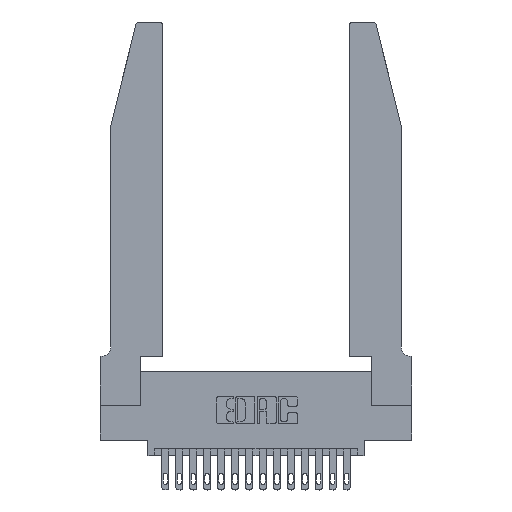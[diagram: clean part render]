
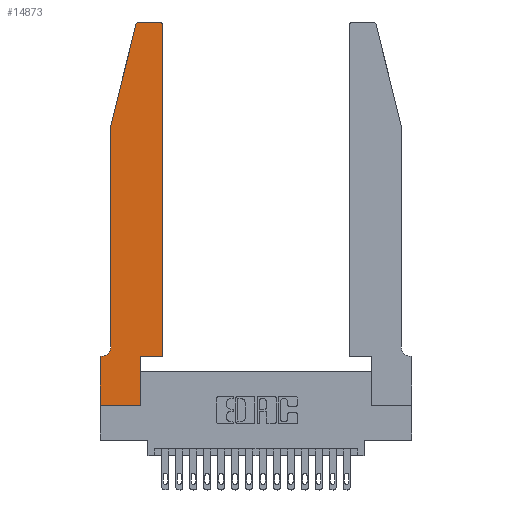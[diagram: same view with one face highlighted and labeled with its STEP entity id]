
A CAD part, top view. The second image highlights one B-rep face of the part: STEP entity #14873.
In plain terms, the highlighted planar face has unit normal (0, 0, 1).
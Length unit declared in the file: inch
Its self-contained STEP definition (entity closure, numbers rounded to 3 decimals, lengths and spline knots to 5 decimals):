
#14 = ORIENTED_EDGE ( 'NONE', *, *, #12326, .T. ) ;
#143 = LINE ( 'NONE', #4160, #15721 ) ;
#217 = VERTEX_POINT ( 'NONE', #1713 ) ;
#735 = EDGE_CURVE ( 'NONE', #17739, #10834, #6813, .T. ) ;
#847 = VERTEX_POINT ( 'NONE', #17734 ) ;
#908 = VECTOR ( 'NONE', #5271, 39.37008 ) ;
#1430 = LINE ( 'NONE', #10283, #4965 ) ;
#1468 = VERTEX_POINT ( 'NONE', #16891 ) ;
#1713 = CARTESIAN_POINT ( 'NONE',  ( 0.2865, 0., 0.37 ) ) ;
#1727 = LINE ( 'NONE', #3205, #10289 ) ;
#2108 = ORIENTED_EDGE ( 'NONE', *, *, #10911, .T. ) ;
#2228 = CARTESIAN_POINT ( 'NONE',  ( 0.4505, 0.35, 0.37 ) ) ;
#2345 = ORIENTED_EDGE ( 'NONE', *, *, #735, .T. ) ;
#2413 = EDGE_CURVE ( 'NONE', #13488, #6220, #143, .T. ) ;
#2883 = ORIENTED_EDGE ( 'NONE', *, *, #5031, .T. ) ;
#3011 = EDGE_CURVE ( 'NONE', #11351, #13488, #18828, .T. ) ;
#3040 = EDGE_CURVE ( 'NONE', #6220, #1468, #1727, .T. ) ;
#3059 = VERTEX_POINT ( 'NONE', #13959 ) ;
#3205 = CARTESIAN_POINT ( 'NONE',  ( 0.0755, 2., 0.37 ) ) ;
#3376 = EDGE_CURVE ( 'NONE', #16136, #847, #13085, .T. ) ;
#3773 = DIRECTION ( 'NONE',  ( -1., 0., 0. ) ) ;
#3942 = DIRECTION ( 'NONE',  ( -1., 0., 0. ) ) ;
#4095 = VECTOR ( 'NONE', #14769, 39.37008 ) ;
#4160 = CARTESIAN_POINT ( 'NONE',  ( 0.0755, 2., 0.37 ) ) ;
#4263 = CARTESIAN_POINT ( 'NONE',  ( 0.0755, 2., 0.37 ) ) ;
#4267 = CARTESIAN_POINT ( 'NONE',  ( 0.2865, 0.35, 0.37 ) ) ;
#4414 = ORIENTED_EDGE ( 'NONE', *, *, #9771, .T. ) ;
#4450 = CARTESIAN_POINT ( 'NONE',  ( 0., 0., 0.37 ) ) ;
#4965 = VECTOR ( 'NONE', #17643, 39.37008 ) ;
#5031 = EDGE_CURVE ( 'NONE', #1468, #17313, #15899, .T. ) ;
#5211 = CARTESIAN_POINT ( 'NONE',  ( 0.4505, 0.35, 0.37 ) ) ;
#5271 = DIRECTION ( 'NONE',  ( 1., 0., 0. ) ) ;
#5745 = FACE_OUTER_BOUND ( 'NONE', #14162, .T. ) ;
#5766 = CARTESIAN_POINT ( 'NONE',  ( 0.4205, 2.72, 0.37 ) ) ;
#6220 = VERTEX_POINT ( 'NONE', #4263 ) ;
#6303 = DIRECTION ( 'NONE',  ( 1., 0., 0. ) ) ;
#6436 = LINE ( 'NONE', #4267, #4095 ) ;
#6813 = LINE ( 'NONE', #2228, #908 ) ;
#6867 = CARTESIAN_POINT ( 'NONE',  ( 0.25487, 2.72718, 0.37 ) ) ;
#6932 = CARTESIAN_POINT ( 'NONE',  ( 0.0055, 0.42, 0.37 ) ) ;
#7708 = VECTOR ( 'NONE', #3942, 39.37008 ) ;
#7959 = CARTESIAN_POINT ( 'NONE',  ( 0.284, 2.72, 0.37 ) ) ;
#8026 = DIRECTION ( 'NONE',  ( 0., -1., 0. ) ) ;
#8660 = DIRECTION ( 'NONE',  ( 0., 1., 0. ) ) ;
#8820 = DIRECTION ( 'NONE',  ( 0., 0., 1. ) ) ;
#8932 = VERTEX_POINT ( 'NONE', #14517 ) ;
#9090 = VECTOR ( 'NONE', #8660, 39.37008 ) ;
#9267 = CARTESIAN_POINT ( 'NONE',  ( 0.4505, 0.35, 0.37 ) ) ;
#9771 = EDGE_CURVE ( 'NONE', #3059, #217, #13580, .T. ) ;
#9833 = DIRECTION ( 'NONE',  ( 0., 0., -1. ) ) ;
#10019 = ORIENTED_EDGE ( 'NONE', *, *, #3040, .T. ) ;
#10212 = PLANE ( 'NONE',  #14861 ) ;
#10280 = DIRECTION ( 'NONE',  ( 0., 0., 1. ) ) ;
#10283 = CARTESIAN_POINT ( 'NONE',  ( 0., 0., 0.37 ) ) ;
#10289 = VECTOR ( 'NONE', #8026, 39.37008 ) ;
#10834 = VERTEX_POINT ( 'NONE', #9267 ) ;
#10911 = EDGE_CURVE ( 'NONE', #10834, #16136, #16198, .T. ) ;
#11351 = VERTEX_POINT ( 'NONE', #15103 ) ;
#11529 = DIRECTION ( 'NONE',  ( 1., 0., 0. ) ) ;
#11720 = LINE ( 'NONE', #17442, #7708 ) ;
#11787 = CARTESIAN_POINT ( 'NONE',  ( 0., 0.35, 0.37 ) ) ;
#12030 = DIRECTION ( 'NONE',  ( 1., 0., 0. ) ) ;
#12326 = EDGE_CURVE ( 'NONE', #17313, #8932, #16265, .T. ) ;
#12334 = ORIENTED_EDGE ( 'NONE', *, *, #3011, .T. ) ;
#12375 = AXIS2_PLACEMENT_3D ( 'NONE', #7959, #13832, #6303 ) ;
#13019 = EDGE_CURVE ( 'NONE', #847, #11351, #11720, .T. ) ;
#13053 = CARTESIAN_POINT ( 'NONE',  ( 0.0055, 0.35, 0.37 ) ) ;
#13057 = DIRECTION ( 'NONE',  ( -1., 0., 0. ) ) ;
#13085 = CIRCLE ( 'NONE', #15807, 0.03 ) ;
#13112 = VECTOR ( 'NONE', #12030, 39.37008 ) ;
#13351 = DIRECTION ( 'NONE',  ( 1., 0., 0. ) ) ;
#13488 = VERTEX_POINT ( 'NONE', #6867 ) ;
#13580 = LINE ( 'NONE', #4450, #13112 ) ;
#13653 = AXIS2_PLACEMENT_3D ( 'NONE', #6932, #9833, #13057 ) ;
#13832 = DIRECTION ( 'NONE',  ( 0., 0., 1. ) ) ;
#13959 = CARTESIAN_POINT ( 'NONE',  ( 0., 0., 0.37 ) ) ;
#14162 = EDGE_LOOP ( 'NONE', ( #16078, #12334, #19087, #10019, #2883, #14, #15025, #4414, #15898, #2345, #2108, #16089 ) ) ;
#14208 = CARTESIAN_POINT ( 'NONE',  ( 0.2865, 0.35, 0.37 ) ) ;
#14517 = CARTESIAN_POINT ( 'NONE',  ( 0., 0.35, 0.37 ) ) ;
#14769 = DIRECTION ( 'NONE',  ( 0., 1., 0. ) ) ;
#14785 = EDGE_CURVE ( 'NONE', #217, #17739, #6436, .T. ) ;
#14861 = AXIS2_PLACEMENT_3D ( 'NONE', #11787, #8820, #11529 ) ;
#14873 = ADVANCED_FACE ( 'NONE', ( #5745 ), #10212, .T. ) ;
#15025 = ORIENTED_EDGE ( 'NONE', *, *, #15849, .T. ) ;
#15103 = CARTESIAN_POINT ( 'NONE',  ( 0.284, 2.75, 0.37 ) ) ;
#15335 = CARTESIAN_POINT ( 'NONE',  ( 0.4505, 2.72, 0.37 ) ) ;
#15721 = VECTOR ( 'NONE', #17609, 39.37008 ) ;
#15800 = CARTESIAN_POINT ( 'NONE',  ( 0.0755, 0.35, 0.37 ) ) ;
#15807 = AXIS2_PLACEMENT_3D ( 'NONE', #5766, #10280, #13351 ) ;
#15849 = EDGE_CURVE ( 'NONE', #8932, #3059, #1430, .T. ) ;
#15898 = ORIENTED_EDGE ( 'NONE', *, *, #14785, .T. ) ;
#15899 = CIRCLE ( 'NONE', #13653, 0.07 ) ;
#16078 = ORIENTED_EDGE ( 'NONE', *, *, #13019, .T. ) ;
#16089 = ORIENTED_EDGE ( 'NONE', *, *, #3376, .T. ) ;
#16136 = VERTEX_POINT ( 'NONE', #15335 ) ;
#16198 = LINE ( 'NONE', #5211, #9090 ) ;
#16265 = LINE ( 'NONE', #15800, #19366 ) ;
#16891 = CARTESIAN_POINT ( 'NONE',  ( 0.0755, 0.42, 0.37 ) ) ;
#17313 = VERTEX_POINT ( 'NONE', #13053 ) ;
#17442 = CARTESIAN_POINT ( 'NONE',  ( 0.2605, 2.75, 0.37 ) ) ;
#17609 = DIRECTION ( 'NONE',  ( -0.239, -0.971, 0. ) ) ;
#17643 = DIRECTION ( 'NONE',  ( 0., -1., 0. ) ) ;
#17734 = CARTESIAN_POINT ( 'NONE',  ( 0.4205, 2.75, 0.37 ) ) ;
#17739 = VERTEX_POINT ( 'NONE', #14208 ) ;
#18828 = CIRCLE ( 'NONE', #12375, 0.03 ) ;
#19087 = ORIENTED_EDGE ( 'NONE', *, *, #2413, .T. ) ;
#19366 = VECTOR ( 'NONE', #3773, 39.37008 ) ;
